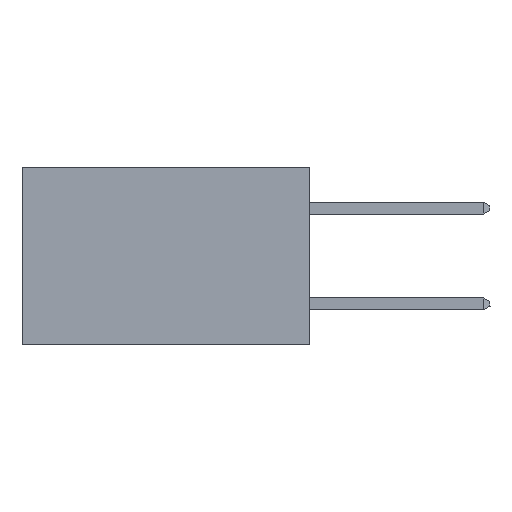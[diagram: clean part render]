
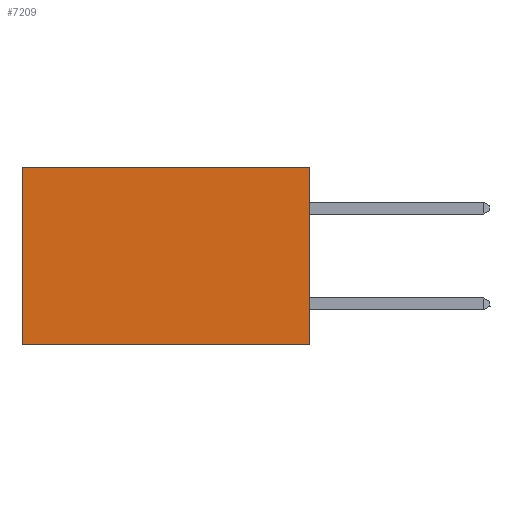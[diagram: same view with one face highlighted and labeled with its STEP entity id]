
A CAD part, left-side view. The second image highlights one B-rep face of the part: STEP entity #7209.
In plain terms, the highlighted planar face has unit normal (-1, 0, 0).
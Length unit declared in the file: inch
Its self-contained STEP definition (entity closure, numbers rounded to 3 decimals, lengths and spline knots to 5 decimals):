
#500 = DIRECTION ( 'NONE',  ( 0., 0., -1. ) ) ;
#669 = AXIS2_PLACEMENT_3D ( 'NONE', #2938, #698, #500 ) ;
#698 = DIRECTION ( 'NONE',  ( 1., 0., 0. ) ) ;
#710 = EDGE_CURVE ( 'NONE', #8145, #17843, #12169, .T. ) ;
#1343 = ORIENTED_EDGE ( 'NONE', *, *, #2274, .T. ) ;
#1485 = EDGE_CURVE ( 'NONE', #11989, #9337, #9202, .T. ) ;
#2038 = LINE ( 'NONE', #13219, #19044 ) ;
#2274 = EDGE_CURVE ( 'NONE', #17843, #9337, #14161, .T. ) ;
#2938 = CARTESIAN_POINT ( 'NONE',  ( 0.2875, 0., 0. ) ) ;
#2969 = ORIENTED_EDGE ( 'NONE', *, *, #1485, .F. ) ;
#3103 = EDGE_CURVE ( 'NONE', #8145, #11989, #2038, .T. ) ;
#3133 = DIRECTION ( 'NONE',  ( 0., 0., -1. ) ) ;
#5637 = CARTESIAN_POINT ( 'NONE',  ( 0.2875, 0.6, -0.37 ) ) ;
#5676 = FACE_OUTER_BOUND ( 'NONE', #11287, .T. ) ;
#6933 = CARTESIAN_POINT ( 'NONE',  ( 0.2875, 0.6, 0. ) ) ;
#7209 = ADVANCED_FACE ( 'NONE', ( #5676 ), #17561, .F. ) ;
#8107 = DIRECTION ( 'NONE',  ( 0., 0., -1. ) ) ;
#8145 = VERTEX_POINT ( 'NONE', #13379 ) ;
#8306 = CARTESIAN_POINT ( 'NONE',  ( 0.2875, 0., -0.37 ) ) ;
#9202 = LINE ( 'NONE', #10777, #13942 ) ;
#9337 = VERTEX_POINT ( 'NONE', #5637 ) ;
#10103 = CARTESIAN_POINT ( 'NONE',  ( 0.2875, 0., 0. ) ) ;
#10777 = CARTESIAN_POINT ( 'NONE',  ( 0.2875, 0., -0.37 ) ) ;
#11287 = EDGE_LOOP ( 'NONE', ( #1343, #2969, #13316, #12421 ) ) ;
#11989 = VERTEX_POINT ( 'NONE', #8306 ) ;
#12169 = LINE ( 'NONE', #10103, #18137 ) ;
#12335 = VECTOR ( 'NONE', #8107, 39.37008 ) ;
#12421 = ORIENTED_EDGE ( 'NONE', *, *, #710, .T. ) ;
#13219 = CARTESIAN_POINT ( 'NONE',  ( 0.2875, 0., 0. ) ) ;
#13316 = ORIENTED_EDGE ( 'NONE', *, *, #3103, .F. ) ;
#13379 = CARTESIAN_POINT ( 'NONE',  ( 0.2875, 0., 0. ) ) ;
#13942 = VECTOR ( 'NONE', #17565, 39.37008 ) ;
#14161 = LINE ( 'NONE', #16664, #12335 ) ;
#15394 = DIRECTION ( 'NONE',  ( 0., 1., 0. ) ) ;
#16664 = CARTESIAN_POINT ( 'NONE',  ( 0.2875, 0.6, 0. ) ) ;
#17561 = PLANE ( 'NONE',  #669 ) ;
#17565 = DIRECTION ( 'NONE',  ( 0., 1., 0. ) ) ;
#17843 = VERTEX_POINT ( 'NONE', #6933 ) ;
#18137 = VECTOR ( 'NONE', #15394, 39.37008 ) ;
#19044 = VECTOR ( 'NONE', #3133, 39.37008 ) ;
